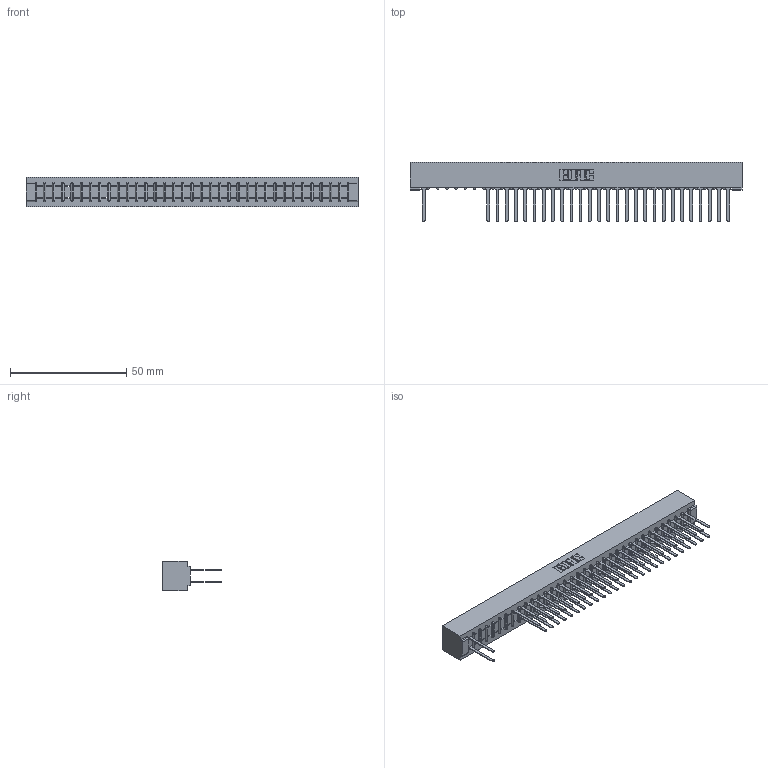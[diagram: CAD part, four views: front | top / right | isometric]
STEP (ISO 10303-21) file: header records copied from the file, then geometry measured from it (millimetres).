
FILE_DESCRIPTION (( 'STEP AP203' ), '1' );
FILE_NAME ('307-068-542-201.STEP', '2018-08-06T12:03:57', ( '' ), ( '' ), 'SwSTEP 2.0', 'SolidWorks 2016', '' );
FILE_SCHEMA (( 'CONFIG_CONTROL_DESIGN' ));
Length unit declared in the file: inch
Products named in the file (3): 307-068-542-201; 307 Part_No Mounting Lugs; 307-290-001_542
Assembly tree (56 placements, depth 2):
  307-068-542-201
    307 Part_No Mounting Lugs
    307-290-001_542  x55
Bounding box: 142.6 x 25.43 x 12.7 mm (x, y, z)
Volume: 15696 mm3; surface area: 19452.7 mm2
Topology: 56 solids, 56 shells, 2805 faces, 7865 edges, 5074 vertices
Faces by surface type: plane 1849, cylinder 886, sphere 70
Entity records: 30496 total; most frequent: CARTESIAN_POINT 5041, ORIENTED_EDGE 5006, DIRECTION 4927, EDGE_CURVE 2503, LINE 1919, VECTOR 1919, VERTEX_POINT 1618, AXIS2_PLACEMENT_3D 1504
